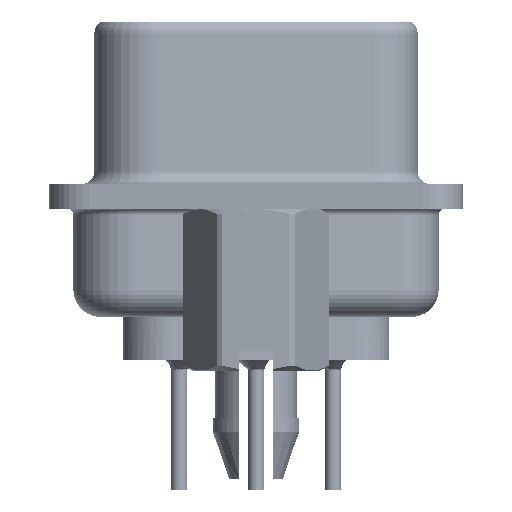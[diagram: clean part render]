
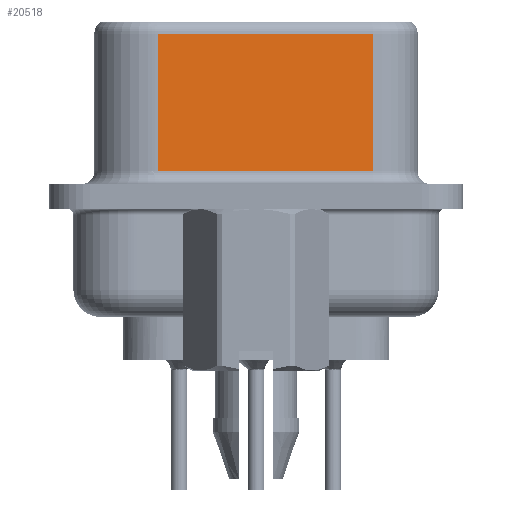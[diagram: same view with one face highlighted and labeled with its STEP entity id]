
A CAD part, left-side view. The second image highlights one B-rep face of the part: STEP entity #20518.
In plain terms, the highlighted planar face has unit normal (-0.985, -0.174, 0).
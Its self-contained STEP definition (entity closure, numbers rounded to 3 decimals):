
#1083 = ORIENTED_EDGE ( 'NONE', *, *, #22715, .F. ) ;
#3153 = CARTESIAN_POINT ( 'NONE',  ( 3.73, 3.628, 6.52 ) ) ;
#3249 = EDGE_CURVE ( 'NONE', #12156, #11206, #14149, .T. ) ;
#4051 = LINE ( 'NONE', #6878, #16959 ) ;
#4075 = DIRECTION ( 'NONE',  ( 0., 0., -1. ) ) ;
#5657 = DIRECTION ( 'NONE',  ( -0.174, 0.985, 0. ) ) ;
#6878 = CARTESIAN_POINT ( 'NONE',  ( 5.132, -4.322, 6.02 ) ) ;
#8242 = LINE ( 'NONE', #3153, #33113 ) ;
#8486 = DIRECTION ( 'NONE',  ( 0.985, 0.174, 0. ) ) ;
#10401 = VERTEX_POINT ( 'NONE', #13634 ) ;
#10520 = VERTEX_POINT ( 'NONE', #11201 ) ;
#11201 = CARTESIAN_POINT ( 'NONE',  ( 5.132, -4.322, 6.02 ) ) ;
#11206 = VERTEX_POINT ( 'NONE', #33096 ) ;
#11747 = EDGE_CURVE ( 'NONE', #10401, #12156, #8242, .T. ) ;
#11971 = ORIENTED_EDGE ( 'NONE', *, *, #26784, .T. ) ;
#12156 = VERTEX_POINT ( 'NONE', #19491 ) ;
#13634 = CARTESIAN_POINT ( 'NONE',  ( 3.73, 3.628, 6.02 ) ) ;
#14149 = LINE ( 'NONE', #25620, #16469 ) ;
#14620 = DIRECTION ( 'NONE',  ( 0., 0., -1. ) ) ;
#15102 = ORIENTED_EDGE ( 'NONE', *, *, #11747, .T. ) ;
#15715 = DIRECTION ( 'NONE',  ( -0.174, 0.985, 0. ) ) ;
#16469 = VECTOR ( 'NONE', #34438, 1000. ) ;
#16569 = FACE_OUTER_BOUND ( 'NONE', #16685, .T. ) ;
#16685 = EDGE_LOOP ( 'NONE', ( #1083, #11971, #15102, #37152 ) ) ;
#16959 = VECTOR ( 'NONE', #15715, 1000. ) ;
#19491 = CARTESIAN_POINT ( 'NONE',  ( 3.73, 3.628, 0.95 ) ) ;
#20518 = ADVANCED_FACE ( 'NONE', ( #16569 ), #25596, .F. ) ;
#21573 = CARTESIAN_POINT ( 'NONE',  ( 5.132, -4.322, 6.52 ) ) ;
#22715 = EDGE_CURVE ( 'NONE', #10520, #11206, #29813, .T. ) ;
#25596 = PLANE ( 'NONE',  #32406 ) ;
#25620 = CARTESIAN_POINT ( 'NONE',  ( 5.132, -4.322, 0.95 ) ) ;
#26784 = EDGE_CURVE ( 'NONE', #10520, #10401, #4051, .T. ) ;
#29813 = LINE ( 'NONE', #21573, #32951 ) ;
#32406 = AXIS2_PLACEMENT_3D ( 'NONE', #34412, #8486, #5657 ) ;
#32951 = VECTOR ( 'NONE', #4075, 1000. ) ;
#33096 = CARTESIAN_POINT ( 'NONE',  ( 5.132, -4.322, 0.95 ) ) ;
#33113 = VECTOR ( 'NONE', #14620, 1000. ) ;
#34412 = CARTESIAN_POINT ( 'NONE',  ( 5.132, -4.322, 6.52 ) ) ;
#34438 = DIRECTION ( 'NONE',  ( 0.174, -0.985, 0. ) ) ;
#37152 = ORIENTED_EDGE ( 'NONE', *, *, #3249, .T. ) ;
